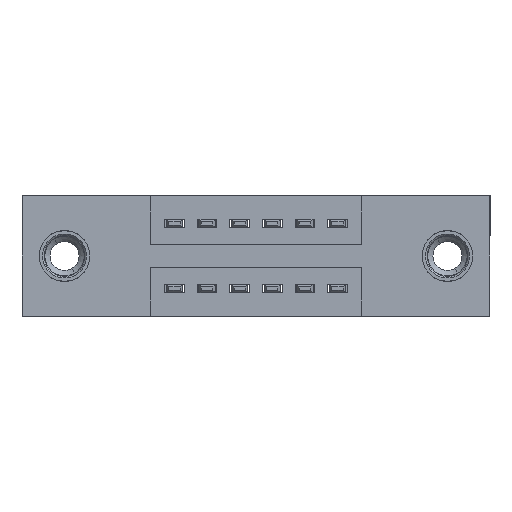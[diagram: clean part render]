
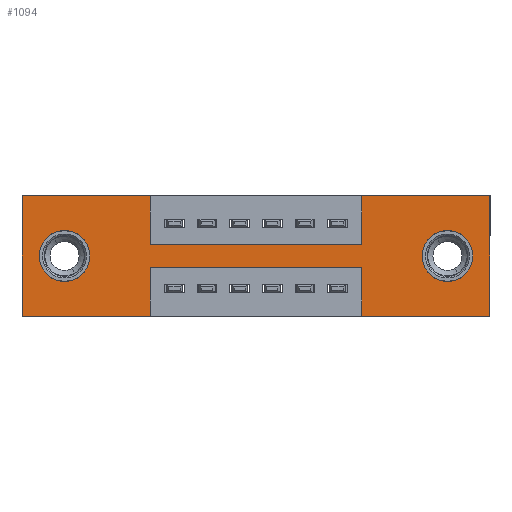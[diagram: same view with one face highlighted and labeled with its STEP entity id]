
A CAD part, front view. The second image highlights one B-rep face of the part: STEP entity #1094.
In plain terms, the highlighted planar face has unit normal (0, -1, 0).
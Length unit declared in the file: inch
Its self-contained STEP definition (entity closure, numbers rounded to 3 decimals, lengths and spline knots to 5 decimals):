
#181 = FACE_OUTER_BOUND ( 'NONE', #3460, .T. ) ;
#343 = CARTESIAN_POINT ( 'NONE',  ( 0.13, 0., -0.107 ) ) ;
#358 = ORIENTED_EDGE ( 'NONE', *, *, #2442, .F. ) ;
#511 = VERTEX_POINT ( 'NONE', #7501 ) ;
#517 = CARTESIAN_POINT ( 'NONE',  ( 0.3925, 0., -0.37 ) ) ;
#565 = LINE ( 'NONE', #2394, #5038 ) ;
#571 = DIRECTION ( 'NONE',  ( 0., 0., 1. ) ) ;
#681 = LINE ( 'NONE', #6669, #2926 ) ;
#690 = CARTESIAN_POINT ( 'NONE',  ( 1.0425, 0., -0.37 ) ) ;
#784 = EDGE_CURVE ( 'NONE', #3086, #9394, #9845, .T. ) ;
#891 = EDGE_CURVE ( 'NONE', #8082, #1015, #11489, .T. ) ;
#929 = CARTESIAN_POINT ( 'NONE',  ( 1.0425, 0., 0. ) ) ;
#1015 = VERTEX_POINT ( 'NONE', #10101 ) ;
#1094 = ADVANCED_FACE ( 'NONE', ( #6303, #5877, #181 ), #3178, .T. ) ;
#1228 = ORIENTED_EDGE ( 'NONE', *, *, #9489, .F. ) ;
#1312 = CIRCLE ( 'NONE', #6050, 0.078 ) ;
#1336 = VECTOR ( 'NONE', #8088, 39.37008 ) ;
#1387 = EDGE_CURVE ( 'NONE', #1905, #511, #11480, .T. ) ;
#1432 = ORIENTED_EDGE ( 'NONE', *, *, #3801, .F. ) ;
#1486 = ORIENTED_EDGE ( 'NONE', *, *, #3922, .F. ) ;
#1645 = LINE ( 'NONE', #690, #2787 ) ;
#1697 = DIRECTION ( 'NONE',  ( 0., 0., 1. ) ) ;
#1719 = LINE ( 'NONE', #4337, #4391 ) ;
#1731 = EDGE_CURVE ( 'NONE', #9394, #11125, #11323, .T. ) ;
#1737 = CARTESIAN_POINT ( 'NONE',  ( 0., 0., 0. ) ) ;
#1768 = DIRECTION ( 'NONE',  ( 0., 1., 0. ) ) ;
#1797 = LINE ( 'NONE', #6021, #10749 ) ;
#1812 = ORIENTED_EDGE ( 'NONE', *, *, #1731, .F. ) ;
#1905 = VERTEX_POINT ( 'NONE', #1737 ) ;
#1930 = CARTESIAN_POINT ( 'NONE',  ( 1.435, 0., 0. ) ) ;
#2054 = VECTOR ( 'NONE', #5026, 39.37008 ) ;
#2064 = VERTEX_POINT ( 'NONE', #6505 ) ;
#2104 = ORIENTED_EDGE ( 'NONE', *, *, #11008, .T. ) ;
#2394 = CARTESIAN_POINT ( 'NONE',  ( 0., 0., 0. ) ) ;
#2442 = EDGE_CURVE ( 'NONE', #511, #8092, #1797, .T. ) ;
#2462 = DIRECTION ( 'NONE',  ( 0., 1., 0. ) ) ;
#2579 = CARTESIAN_POINT ( 'NONE',  ( 1.305, 0., -0.185 ) ) ;
#2750 = EDGE_CURVE ( 'NONE', #2064, #10912, #681, .T. ) ;
#2757 = CARTESIAN_POINT ( 'NONE',  ( 0.3925, 0., -0.15 ) ) ;
#2766 = CIRCLE ( 'NONE', #8459, 0.078 ) ;
#2787 = VECTOR ( 'NONE', #1697, 39.37008 ) ;
#2801 = VERTEX_POINT ( 'NONE', #4752 ) ;
#2926 = VECTOR ( 'NONE', #8346, 39.37008 ) ;
#2981 = AXIS2_PLACEMENT_3D ( 'NONE', #4198, #2462, #6039 ) ;
#3008 = DIRECTION ( 'NONE',  ( 0., 0., 1. ) ) ;
#3086 = VERTEX_POINT ( 'NONE', #8137 ) ;
#3104 = CARTESIAN_POINT ( 'NONE',  ( 1.0425, 0., -0.15 ) ) ;
#3178 = PLANE ( 'NONE',  #11346 ) ;
#3209 = ORIENTED_EDGE ( 'NONE', *, *, #9166, .F. ) ;
#3277 = VERTEX_POINT ( 'NONE', #3104 ) ;
#3460 = EDGE_LOOP ( 'NONE', ( #5943, #9716, #1228, #3668, #3209, #1432, #1486, #11025, #358, #11080, #5496, #1812 ) ) ;
#3466 = LINE ( 'NONE', #5729, #6096 ) ;
#3668 = ORIENTED_EDGE ( 'NONE', *, *, #2750, .F. ) ;
#3801 = EDGE_CURVE ( 'NONE', #2801, #7753, #3466, .T. ) ;
#3922 = EDGE_CURVE ( 'NONE', #3277, #2801, #8614, .T. ) ;
#4198 = CARTESIAN_POINT ( 'NONE',  ( 1.305, 0., -0.185 ) ) ;
#4337 = CARTESIAN_POINT ( 'NONE',  ( 0.3925, 0., -0.15 ) ) ;
#4391 = VECTOR ( 'NONE', #5318, 39.37008 ) ;
#4532 = AXIS2_PLACEMENT_3D ( 'NONE', #8560, #8516, #571 ) ;
#4752 = CARTESIAN_POINT ( 'NONE',  ( 1.0425, 0., 0. ) ) ;
#4920 = CARTESIAN_POINT ( 'NONE',  ( 0., 0., -0.37 ) ) ;
#5011 = CARTESIAN_POINT ( 'NONE',  ( 0.13, 0., -0.263 ) ) ;
#5026 = DIRECTION ( 'NONE',  ( 0., 0., -1. ) ) ;
#5038 = VECTOR ( 'NONE', #10485, 39.37008 ) ;
#5093 = DIRECTION ( 'NONE',  ( -1., 0., 0. ) ) ;
#5172 = CARTESIAN_POINT ( 'NONE',  ( 0., 0., -0.37 ) ) ;
#5202 = CARTESIAN_POINT ( 'NONE',  ( 0.3925, 0., -0.22 ) ) ;
#5247 = VECTOR ( 'NONE', #7085, 39.37008 ) ;
#5318 = DIRECTION ( 'NONE',  ( 1., 0., 0. ) ) ;
#5413 = EDGE_CURVE ( 'NONE', #8092, #3277, #1719, .T. ) ;
#5496 = ORIENTED_EDGE ( 'NONE', *, *, #6247, .F. ) ;
#5679 = LINE ( 'NONE', #7570, #2054 ) ;
#5729 = CARTESIAN_POINT ( 'NONE',  ( 0., 0., 0. ) ) ;
#5802 = DIRECTION ( 'NONE',  ( 0., -1., 0. ) ) ;
#5877 = FACE_BOUND ( 'NONE', #9581, .T. ) ;
#5929 = ORIENTED_EDGE ( 'NONE', *, *, #891, .T. ) ;
#5943 = ORIENTED_EDGE ( 'NONE', *, *, #784, .F. ) ;
#6021 = CARTESIAN_POINT ( 'NONE',  ( 0.3925, 0., 0. ) ) ;
#6039 = DIRECTION ( 'NONE',  ( 0., 0., -1. ) ) ;
#6050 = AXIS2_PLACEMENT_3D ( 'NONE', #10738, #10091, #3008 ) ;
#6096 = VECTOR ( 'NONE', #7846, 39.37008 ) ;
#6207 = CARTESIAN_POINT ( 'NONE',  ( 1.305, 0., -0.263 ) ) ;
#6247 = EDGE_CURVE ( 'NONE', #11125, #1905, #565, .T. ) ;
#6303 = FACE_BOUND ( 'NONE', #10846, .T. ) ;
#6477 = DIRECTION ( 'NONE',  ( 1., 0., 0. ) ) ;
#6505 = CARTESIAN_POINT ( 'NONE',  ( 1.435, 0., -0.37 ) ) ;
#6669 = CARTESIAN_POINT ( 'NONE',  ( 0., 0., -0.37 ) ) ;
#7085 = DIRECTION ( 'NONE',  ( -1., 0., 0. ) ) ;
#7211 = LINE ( 'NONE', #5202, #5247 ) ;
#7259 = CARTESIAN_POINT ( 'NONE',  ( 1.0425, 0., -0.37 ) ) ;
#7501 = CARTESIAN_POINT ( 'NONE',  ( 0.3925, 0., 0. ) ) ;
#7570 = CARTESIAN_POINT ( 'NONE',  ( 1.435, 0., 0. ) ) ;
#7645 = VERTEX_POINT ( 'NONE', #5011 ) ;
#7753 = VERTEX_POINT ( 'NONE', #1930 ) ;
#7814 = DIRECTION ( 'NONE',  ( 0., 0., -1. ) ) ;
#7846 = DIRECTION ( 'NONE',  ( 1., 0., 0. ) ) ;
#8082 = VERTEX_POINT ( 'NONE', #6207 ) ;
#8088 = DIRECTION ( 'NONE',  ( 0., 0., 1. ) ) ;
#8092 = VERTEX_POINT ( 'NONE', #2757 ) ;
#8137 = CARTESIAN_POINT ( 'NONE',  ( 0.3925, 0., -0.22 ) ) ;
#8346 = DIRECTION ( 'NONE',  ( -1., 0., 0. ) ) ;
#8459 = AXIS2_PLACEMENT_3D ( 'NONE', #2579, #1768, #11426 ) ;
#8516 = DIRECTION ( 'NONE',  ( 0., 1., 0. ) ) ;
#8560 = CARTESIAN_POINT ( 'NONE',  ( 0.13, 0., -0.185 ) ) ;
#8614 = LINE ( 'NONE', #929, #1336 ) ;
#8766 = DIRECTION ( 'NONE',  ( 0., 0., -1. ) ) ;
#8968 = VECTOR ( 'NONE', #5093, 39.37008 ) ;
#9107 = EDGE_CURVE ( 'NONE', #9271, #7645, #10864, .T. ) ;
#9166 = EDGE_CURVE ( 'NONE', #7753, #2064, #5679, .T. ) ;
#9184 = VERTEX_POINT ( 'NONE', #11253 ) ;
#9271 = VERTEX_POINT ( 'NONE', #343 ) ;
#9394 = VERTEX_POINT ( 'NONE', #517 ) ;
#9401 = VECTOR ( 'NONE', #6477, 39.37008 ) ;
#9489 = EDGE_CURVE ( 'NONE', #10912, #9184, #1645, .T. ) ;
#9581 = EDGE_LOOP ( 'NONE', ( #11525, #2104 ) ) ;
#9716 = ORIENTED_EDGE ( 'NONE', *, *, #10199, .F. ) ;
#9845 = LINE ( 'NONE', #10237, #11343 ) ;
#10061 = CARTESIAN_POINT ( 'NONE',  ( 0., 0., 0. ) ) ;
#10091 = DIRECTION ( 'NONE',  ( 0., 1., 0. ) ) ;
#10101 = CARTESIAN_POINT ( 'NONE',  ( 1.305, 0., -0.107 ) ) ;
#10162 = EDGE_CURVE ( 'NONE', #1015, #8082, #2766, .T. ) ;
#10199 = EDGE_CURVE ( 'NONE', #9184, #3086, #7211, .T. ) ;
#10237 = CARTESIAN_POINT ( 'NONE',  ( 0.3925, 0., -0.37 ) ) ;
#10324 = DIRECTION ( 'NONE',  ( 0., 0., -1. ) ) ;
#10458 = CARTESIAN_POINT ( 'NONE',  ( 0., 0., -0.37 ) ) ;
#10485 = DIRECTION ( 'NONE',  ( 0., 0., 1. ) ) ;
#10738 = CARTESIAN_POINT ( 'NONE',  ( 0.13, 0., -0.185 ) ) ;
#10749 = VECTOR ( 'NONE', #7814, 39.37008 ) ;
#10846 = EDGE_LOOP ( 'NONE', ( #11537, #5929 ) ) ;
#10864 = CIRCLE ( 'NONE', #4532, 0.078 ) ;
#10912 = VERTEX_POINT ( 'NONE', #7259 ) ;
#11008 = EDGE_CURVE ( 'NONE', #7645, #9271, #1312, .T. ) ;
#11025 = ORIENTED_EDGE ( 'NONE', *, *, #5413, .F. ) ;
#11080 = ORIENTED_EDGE ( 'NONE', *, *, #1387, .F. ) ;
#11125 = VERTEX_POINT ( 'NONE', #10458 ) ;
#11253 = CARTESIAN_POINT ( 'NONE',  ( 1.0425, 0., -0.22 ) ) ;
#11323 = LINE ( 'NONE', #5172, #8968 ) ;
#11343 = VECTOR ( 'NONE', #8766, 39.37008 ) ;
#11346 = AXIS2_PLACEMENT_3D ( 'NONE', #4920, #5802, #10324 ) ;
#11426 = DIRECTION ( 'NONE',  ( 0., 0., -1. ) ) ;
#11480 = LINE ( 'NONE', #10061, #9401 ) ;
#11489 = CIRCLE ( 'NONE', #2981, 0.078 ) ;
#11525 = ORIENTED_EDGE ( 'NONE', *, *, #9107, .T. ) ;
#11537 = ORIENTED_EDGE ( 'NONE', *, *, #10162, .T. ) ;
